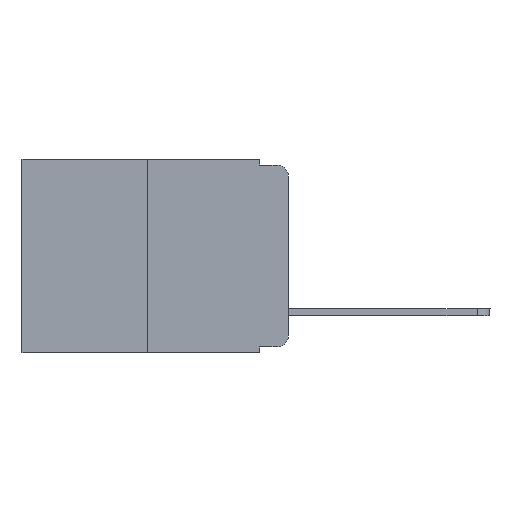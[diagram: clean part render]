
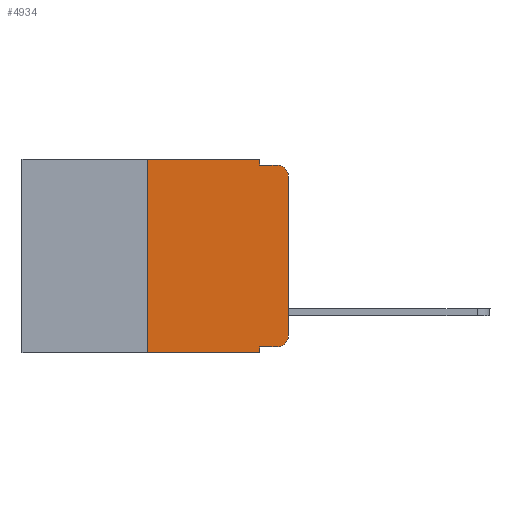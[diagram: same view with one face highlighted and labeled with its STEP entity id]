
A CAD part, left-side view. The second image highlights one B-rep face of the part: STEP entity #4934.
In plain terms, the highlighted planar face has unit normal (-1, 0, 0).
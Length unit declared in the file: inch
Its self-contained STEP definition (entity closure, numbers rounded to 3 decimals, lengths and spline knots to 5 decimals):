
#148 = ORIENTED_EDGE ( 'NONE', *, *, #9531, .T. ) ;
#152 = CARTESIAN_POINT ( 'NONE',  ( 0., 0.051, 0. ) ) ;
#325 = ORIENTED_EDGE ( 'NONE', *, *, #8346, .T. ) ;
#730 = VECTOR ( 'NONE', #7515, 39.37008 ) ;
#780 = DIRECTION ( 'NONE',  ( -1., 0., 0. ) ) ;
#1548 = EDGE_CURVE ( 'NONE', #5145, #7525, #3221, .T. ) ;
#1749 = CARTESIAN_POINT ( 'NONE',  ( 0., 0.473, -0.343 ) ) ;
#1771 = CIRCLE ( 'NONE', #4995, 0.02 ) ;
#1815 = DIRECTION ( 'NONE',  ( 1., 0., 0. ) ) ;
#1973 = CARTESIAN_POINT ( 'NONE',  ( 0., 0., 0. ) ) ;
#2015 = ORIENTED_EDGE ( 'NONE', *, *, #6148, .F. ) ;
#2109 = ORIENTED_EDGE ( 'NONE', *, *, #8577, .F. ) ;
#2160 = CARTESIAN_POINT ( 'NONE',  ( 0., 0.051, 0. ) ) ;
#2311 = VECTOR ( 'NONE', #3371, 39.37008 ) ;
#2566 = LINE ( 'NONE', #6710, #730 ) ;
#2941 = CARTESIAN_POINT ( 'NONE',  ( 0., 0.25, 0. ) ) ;
#3147 = VERTEX_POINT ( 'NONE', #9357 ) ;
#3221 = LINE ( 'NONE', #6783, #10166 ) ;
#3252 = DIRECTION ( 'NONE',  ( 0., 0., -1. ) ) ;
#3279 = EDGE_CURVE ( 'NONE', #4306, #3147, #6726, .T. ) ;
#3286 = LINE ( 'NONE', #1749, #5840 ) ;
#3321 = EDGE_CURVE ( 'NONE', #10061, #10648, #1771, .T. ) ;
#3331 = VECTOR ( 'NONE', #6080, 39.37008 ) ;
#3371 = DIRECTION ( 'NONE',  ( 0., 0., -1. ) ) ;
#3631 = ORIENTED_EDGE ( 'NONE', *, *, #4571, .F. ) ;
#4027 = CARTESIAN_POINT ( 'NONE',  ( 0., 0.051, -0.343 ) ) ;
#4028 = ORIENTED_EDGE ( 'NONE', *, *, #1548, .F. ) ;
#4173 = DIRECTION ( 'NONE',  ( 0., -1., 0. ) ) ;
#4306 = VERTEX_POINT ( 'NONE', #6092 ) ;
#4413 = LINE ( 'NONE', #2160, #2311 ) ;
#4571 = EDGE_CURVE ( 'NONE', #4306, #10224, #5423, .T. ) ;
#4644 = CARTESIAN_POINT ( 'NONE',  ( 0., 0.25, 0. ) ) ;
#4645 = CARTESIAN_POINT ( 'NONE',  ( 0., 0.02, -0.01 ) ) ;
#4703 = EDGE_CURVE ( 'NONE', #7525, #8913, #4413, .T. ) ;
#4934 = ADVANCED_FACE ( 'NONE', ( #8375 ), #5433, .F. ) ;
#4995 = AXIS2_PLACEMENT_3D ( 'NONE', #7984, #780, #6278 ) ;
#5001 = ORIENTED_EDGE ( 'NONE', *, *, #3279, .T. ) ;
#5045 = CARTESIAN_POINT ( 'NONE',  ( 0., 0.051, -0.333 ) ) ;
#5145 = VERTEX_POINT ( 'NONE', #2941 ) ;
#5423 = LINE ( 'NONE', #6922, #10515 ) ;
#5433 = PLANE ( 'NONE',  #7258 ) ;
#5840 = VECTOR ( 'NONE', #10761, 39.37008 ) ;
#5991 = DIRECTION ( 'NONE',  ( -1., 0., 0. ) ) ;
#6055 = EDGE_CURVE ( 'NONE', #11094, #10061, #10071, .T. ) ;
#6074 = ORIENTED_EDGE ( 'NONE', *, *, #3321, .T. ) ;
#6080 = DIRECTION ( 'NONE',  ( 0., -1., 0. ) ) ;
#6092 = CARTESIAN_POINT ( 'NONE',  ( 0., 0.051, -0.333 ) ) ;
#6108 = VECTOR ( 'NONE', #10012, 39.37008 ) ;
#6148 = EDGE_CURVE ( 'NONE', #8913, #10648, #2566, .T. ) ;
#6278 = DIRECTION ( 'NONE',  ( 0., 0., -1. ) ) ;
#6438 = VECTOR ( 'NONE', #9141, 39.37008 ) ;
#6710 = CARTESIAN_POINT ( 'NONE',  ( 0., 0.051, -0.01 ) ) ;
#6717 = LINE ( 'NONE', #4644, #6438 ) ;
#6726 = LINE ( 'NONE', #5045, #3331 ) ;
#6783 = CARTESIAN_POINT ( 'NONE',  ( 0., 0.473, 0. ) ) ;
#6922 = CARTESIAN_POINT ( 'NONE',  ( 0., 0.051, 0. ) ) ;
#7004 = AXIS2_PLACEMENT_3D ( 'NONE', #8673, #5991, #3252 ) ;
#7258 = AXIS2_PLACEMENT_3D ( 'NONE', #8212, #1815, #9988 ) ;
#7402 = CIRCLE ( 'NONE', #7004, 0.02 ) ;
#7496 = DIRECTION ( 'NONE',  ( 0., 0., -1. ) ) ;
#7515 = DIRECTION ( 'NONE',  ( 0., -1., 0. ) ) ;
#7525 = VERTEX_POINT ( 'NONE', #152 ) ;
#7822 = CARTESIAN_POINT ( 'NONE',  ( 0., 0.25, -0.343 ) ) ;
#7984 = CARTESIAN_POINT ( 'NONE',  ( 0., 0.02, -0.03 ) ) ;
#8212 = CARTESIAN_POINT ( 'NONE',  ( 0., 0.473, 0. ) ) ;
#8346 = EDGE_CURVE ( 'NONE', #3147, #11094, #7402, .T. ) ;
#8375 = FACE_OUTER_BOUND ( 'NONE', #10251, .T. ) ;
#8577 = EDGE_CURVE ( 'NONE', #9471, #5145, #6717, .T. ) ;
#8673 = CARTESIAN_POINT ( 'NONE',  ( 0., 0.02, -0.313 ) ) ;
#8801 = ORIENTED_EDGE ( 'NONE', *, *, #4703, .F. ) ;
#8913 = VERTEX_POINT ( 'NONE', #11001 ) ;
#9141 = DIRECTION ( 'NONE',  ( 0., 0., 1. ) ) ;
#9357 = CARTESIAN_POINT ( 'NONE',  ( 0., 0.02, -0.333 ) ) ;
#9471 = VERTEX_POINT ( 'NONE', #7822 ) ;
#9531 = EDGE_CURVE ( 'NONE', #9471, #10224, #3286, .T. ) ;
#9988 = DIRECTION ( 'NONE',  ( 0., 0., -1. ) ) ;
#10012 = DIRECTION ( 'NONE',  ( 0., 0., 1. ) ) ;
#10061 = VERTEX_POINT ( 'NONE', #11029 ) ;
#10071 = LINE ( 'NONE', #1973, #6108 ) ;
#10166 = VECTOR ( 'NONE', #4173, 39.37008 ) ;
#10224 = VERTEX_POINT ( 'NONE', #4027 ) ;
#10251 = EDGE_LOOP ( 'NONE', ( #11274, #6074, #2015, #8801, #4028, #2109, #148, #3631, #5001, #325 ) ) ;
#10515 = VECTOR ( 'NONE', #7496, 39.37008 ) ;
#10648 = VERTEX_POINT ( 'NONE', #4645 ) ;
#10761 = DIRECTION ( 'NONE',  ( 0., -1., 0. ) ) ;
#11001 = CARTESIAN_POINT ( 'NONE',  ( 0., 0.051, -0.01 ) ) ;
#11029 = CARTESIAN_POINT ( 'NONE',  ( 0., 0., -0.03 ) ) ;
#11094 = VERTEX_POINT ( 'NONE', #11502 ) ;
#11274 = ORIENTED_EDGE ( 'NONE', *, *, #6055, .T. ) ;
#11502 = CARTESIAN_POINT ( 'NONE',  ( 0., 0., -0.313 ) ) ;
